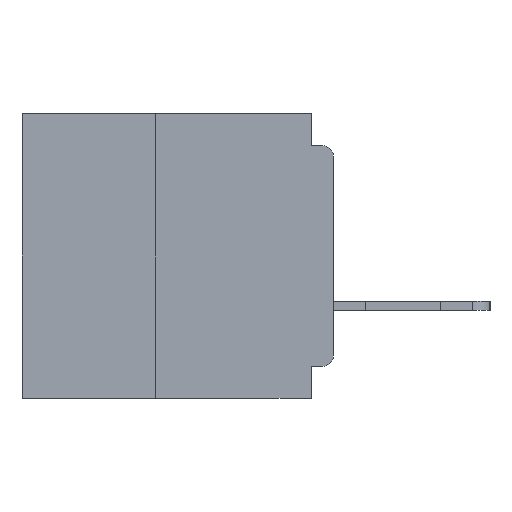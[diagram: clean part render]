
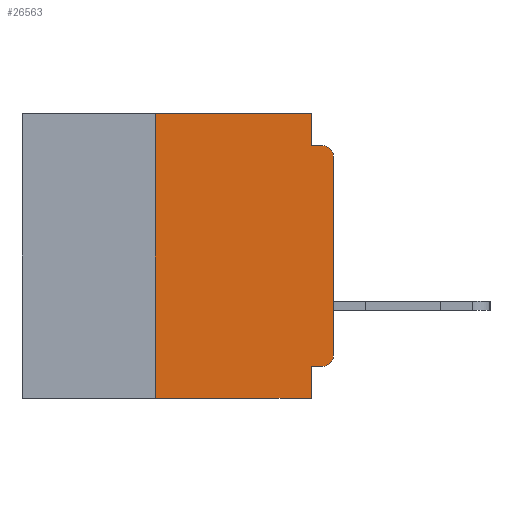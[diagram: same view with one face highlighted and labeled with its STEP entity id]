
A CAD part, left-side view. The second image highlights one B-rep face of the part: STEP entity #26563.
In plain terms, the highlighted planar face has unit normal (-1, 0, 0).
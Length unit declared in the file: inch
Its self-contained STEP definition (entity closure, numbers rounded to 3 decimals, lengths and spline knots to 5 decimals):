
#1688 = AXIS2_PLACEMENT_3D ( 'NONE', #17694, #44914, #21632 ) ;
#1742 = CARTESIAN_POINT ( 'NONE',  ( 0., 0.031, -0.045 ) ) ;
#1964 = CIRCLE ( 'NONE', #46200, 0.015 ) ;
#2061 = VERTEX_POINT ( 'NONE', #23889 ) ;
#2476 = CIRCLE ( 'NONE', #1688, 0.015 ) ;
#3298 = VECTOR ( 'NONE', #29484, 39.37008 ) ;
#3792 = DIRECTION ( 'NONE',  ( 0., -1., 0. ) ) ;
#4180 = CARTESIAN_POINT ( 'NONE',  ( 0., 0.25, -0.4 ) ) ;
#5380 = ORIENTED_EDGE ( 'NONE', *, *, #44810, .T. ) ;
#6045 = CARTESIAN_POINT ( 'NONE',  ( 0., 0.031, -0.4 ) ) ;
#6832 = DIRECTION ( 'NONE',  ( 0., 1., 0. ) ) ;
#6884 = ORIENTED_EDGE ( 'NONE', *, *, #31912, .F. ) ;
#7173 = PLANE ( 'NONE',  #38120 ) ;
#9426 = LINE ( 'NONE', #16837, #39327 ) ;
#9781 = EDGE_CURVE ( 'NONE', #14625, #18370, #9426, .T. ) ;
#9919 = EDGE_CURVE ( 'NONE', #39014, #35287, #1964, .T. ) ;
#10261 = CARTESIAN_POINT ( 'NONE',  ( 0., 0.031, -0.355 ) ) ;
#12740 = CARTESIAN_POINT ( 'NONE',  ( 0., 0., -0.34 ) ) ;
#14625 = VERTEX_POINT ( 'NONE', #28042 ) ;
#14923 = CARTESIAN_POINT ( 'NONE',  ( 0., 0.437, 0. ) ) ;
#15099 = DIRECTION ( 'NONE',  ( 1., 0., 0. ) ) ;
#15474 = EDGE_CURVE ( 'NONE', #31816, #41586, #34517, .T. ) ;
#15973 = LINE ( 'NONE', #30250, #44551 ) ;
#16093 = DIRECTION ( 'NONE',  ( 0., 0., 1. ) ) ;
#16837 = CARTESIAN_POINT ( 'NONE',  ( 0., 0.031, 0. ) ) ;
#17694 = CARTESIAN_POINT ( 'NONE',  ( 0., 0.015, -0.34 ) ) ;
#17843 = CARTESIAN_POINT ( 'NONE',  ( 0., 0.015, -0.06 ) ) ;
#18158 = ORIENTED_EDGE ( 'NONE', *, *, #9781, .F. ) ;
#18370 = VERTEX_POINT ( 'NONE', #1742 ) ;
#19026 = ORIENTED_EDGE ( 'NONE', *, *, #39767, .F. ) ;
#19648 = DIRECTION ( 'NONE',  ( 0., -1., 0. ) ) ;
#20264 = VECTOR ( 'NONE', #19648, 39.37008 ) ;
#21443 = CARTESIAN_POINT ( 'NONE',  ( 0., 0., 0. ) ) ;
#21496 = VECTOR ( 'NONE', #16093, 39.37008 ) ;
#21632 = DIRECTION ( 'NONE',  ( 0., 0., -1. ) ) ;
#21778 = DIRECTION ( 'NONE',  ( 0., 0., -1. ) ) ;
#22540 = LINE ( 'NONE', #23369, #23770 ) ;
#22714 = EDGE_CURVE ( 'NONE', #2061, #33459, #31838, .T. ) ;
#23369 = CARTESIAN_POINT ( 'NONE',  ( 0., 0., -0.045 ) ) ;
#23770 = VECTOR ( 'NONE', #3792, 39.37008 ) ;
#23889 = CARTESIAN_POINT ( 'NONE',  ( 0., 0.25, -0.4 ) ) ;
#24051 = CARTESIAN_POINT ( 'NONE',  ( 0., 0.437, 0. ) ) ;
#25017 = VECTOR ( 'NONE', #39516, 39.37008 ) ;
#25044 = EDGE_CURVE ( 'NONE', #18370, #35287, #22540, .T. ) ;
#25249 = CARTESIAN_POINT ( 'NONE',  ( 0., 0., -0.06 ) ) ;
#25259 = VECTOR ( 'NONE', #29135, 39.37008 ) ;
#26563 = ADVANCED_FACE ( 'NONE', ( #42458 ), #7173, .F. ) ;
#28042 = CARTESIAN_POINT ( 'NONE',  ( 0., 0.031, 0. ) ) ;
#28350 = ORIENTED_EDGE ( 'NONE', *, *, #35965, .T. ) ;
#29135 = DIRECTION ( 'NONE',  ( 0., 0., 1. ) ) ;
#29484 = DIRECTION ( 'NONE',  ( 0., 0., -1. ) ) ;
#30250 = CARTESIAN_POINT ( 'NONE',  ( 0., 0., -0.355 ) ) ;
#31816 = VERTEX_POINT ( 'NONE', #10261 ) ;
#31838 = LINE ( 'NONE', #4180, #21496 ) ;
#31912 = EDGE_CURVE ( 'NONE', #35101, #31816, #15973, .T. ) ;
#33034 = ORIENTED_EDGE ( 'NONE', *, *, #25044, .F. ) ;
#33459 = VERTEX_POINT ( 'NONE', #48280 ) ;
#34033 = EDGE_LOOP ( 'NONE', ( #28350, #48942, #33034, #18158, #19026, #46675, #44307, #42257, #6884, #5380 ) ) ;
#34517 = LINE ( 'NONE', #6045, #3298 ) ;
#35101 = VERTEX_POINT ( 'NONE', #46685 ) ;
#35287 = VERTEX_POINT ( 'NONE', #47853 ) ;
#35965 = EDGE_CURVE ( 'NONE', #42881, #39014, #45913, .T. ) ;
#38120 = AXIS2_PLACEMENT_3D ( 'NONE', #14923, #15099, #42326 ) ;
#38527 = LINE ( 'NONE', #42957, #20264 ) ;
#38670 = CARTESIAN_POINT ( 'NONE',  ( 0., 0.031, -0.4 ) ) ;
#39014 = VERTEX_POINT ( 'NONE', #25249 ) ;
#39327 = VECTOR ( 'NONE', #47974, 39.37008 ) ;
#39516 = DIRECTION ( 'NONE',  ( 0., -1., 0. ) ) ;
#39767 = EDGE_CURVE ( 'NONE', #33459, #14625, #45687, .T. ) ;
#41586 = VERTEX_POINT ( 'NONE', #38670 ) ;
#42257 = ORIENTED_EDGE ( 'NONE', *, *, #15474, .F. ) ;
#42326 = DIRECTION ( 'NONE',  ( 0., 0., -1. ) ) ;
#42458 = FACE_OUTER_BOUND ( 'NONE', #34033, .T. ) ;
#42881 = VERTEX_POINT ( 'NONE', #12740 ) ;
#42957 = CARTESIAN_POINT ( 'NONE',  ( 0., 0.437, -0.4 ) ) ;
#43984 = EDGE_CURVE ( 'NONE', #2061, #41586, #38527, .T. ) ;
#44307 = ORIENTED_EDGE ( 'NONE', *, *, #43984, .T. ) ;
#44551 = VECTOR ( 'NONE', #6832, 39.37008 ) ;
#44810 = EDGE_CURVE ( 'NONE', #35101, #42881, #2476, .T. ) ;
#44914 = DIRECTION ( 'NONE',  ( -1., 0., 0. ) ) ;
#45059 = DIRECTION ( 'NONE',  ( -1., 0., 0. ) ) ;
#45687 = LINE ( 'NONE', #24051, #25017 ) ;
#45913 = LINE ( 'NONE', #21443, #25259 ) ;
#46200 = AXIS2_PLACEMENT_3D ( 'NONE', #17843, #45059, #21778 ) ;
#46675 = ORIENTED_EDGE ( 'NONE', *, *, #22714, .F. ) ;
#46685 = CARTESIAN_POINT ( 'NONE',  ( 0., 0.015, -0.355 ) ) ;
#47853 = CARTESIAN_POINT ( 'NONE',  ( 0., 0.015, -0.045 ) ) ;
#47974 = DIRECTION ( 'NONE',  ( 0., 0., -1. ) ) ;
#48280 = CARTESIAN_POINT ( 'NONE',  ( 0., 0.25, 0. ) ) ;
#48942 = ORIENTED_EDGE ( 'NONE', *, *, #9919, .T. ) ;
